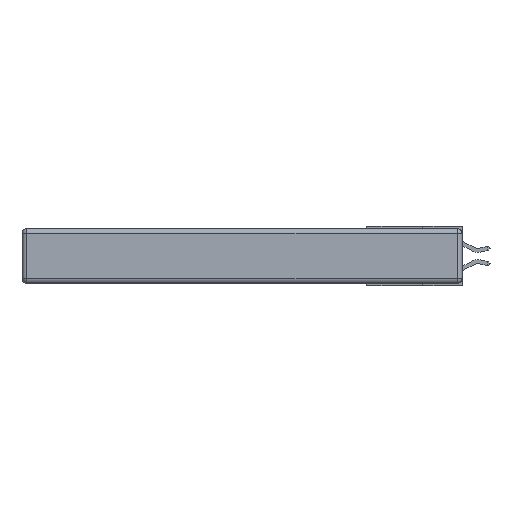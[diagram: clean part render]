
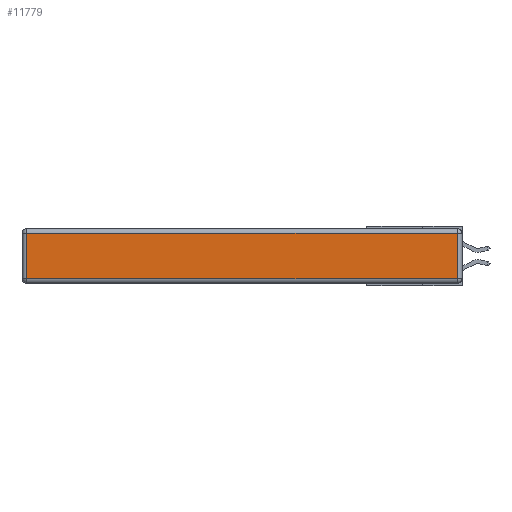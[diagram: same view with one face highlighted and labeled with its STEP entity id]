
A CAD part, left-side view. The second image highlights one B-rep face of the part: STEP entity #11779.
In plain terms, the highlighted planar face has unit normal (-1, 0, 0).
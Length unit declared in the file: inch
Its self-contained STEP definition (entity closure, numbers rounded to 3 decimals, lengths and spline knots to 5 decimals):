
#363 = CARTESIAN_POINT ( 'NONE',  ( 0., 2.72, -0.343 ) ) ;
#680 = ORIENTED_EDGE ( 'NONE', *, *, #1402, .T. ) ;
#689 = PLANE ( 'NONE',  #1484 ) ;
#889 = ORIENTED_EDGE ( 'NONE', *, *, #3025, .T. ) ;
#1402 = EDGE_CURVE ( 'NONE', #5856, #6088, #8198, .T. ) ;
#1484 = AXIS2_PLACEMENT_3D ( 'NONE', #8946, #13952, #6666 ) ;
#1620 = DIRECTION ( 'NONE',  ( 0., 0., -1. ) ) ;
#2012 = ORIENTED_EDGE ( 'NONE', *, *, #2764, .T. ) ;
#2402 = LINE ( 'NONE', #3396, #6455 ) ;
#2764 = EDGE_CURVE ( 'NONE', #6088, #13949, #13641, .T. ) ;
#3025 = EDGE_CURVE ( 'NONE', #13949, #10042, #5143, .T. ) ;
#3141 = VECTOR ( 'NONE', #4670, 39.37008 ) ;
#3396 = CARTESIAN_POINT ( 'NONE',  ( 0., 2.75, -0.03 ) ) ;
#3878 = CARTESIAN_POINT ( 'NONE',  ( 0., 0.03, -0.343 ) ) ;
#4144 = EDGE_LOOP ( 'NONE', ( #2012, #889, #14022, #680 ) ) ;
#4670 = DIRECTION ( 'NONE',  ( 0., -1., 0. ) ) ;
#5143 = LINE ( 'NONE', #3878, #15537 ) ;
#5577 = VECTOR ( 'NONE', #1620, 39.37008 ) ;
#5856 = VERTEX_POINT ( 'NONE', #15125 ) ;
#6088 = VERTEX_POINT ( 'NONE', #9663 ) ;
#6455 = VECTOR ( 'NONE', #14264, 39.37008 ) ;
#6666 = DIRECTION ( 'NONE',  ( 0., 0., 1. ) ) ;
#6733 = CARTESIAN_POINT ( 'NONE',  ( 0., 0.03, -0.03 ) ) ;
#8198 = LINE ( 'NONE', #363, #5577 ) ;
#8717 = FACE_OUTER_BOUND ( 'NONE', #4144, .T. ) ;
#8946 = CARTESIAN_POINT ( 'NONE',  ( 0., 0., -0.343 ) ) ;
#9548 = CARTESIAN_POINT ( 'NONE',  ( 0., 0., -0.313 ) ) ;
#9641 = CARTESIAN_POINT ( 'NONE',  ( 0., 0.03, -0.313 ) ) ;
#9663 = CARTESIAN_POINT ( 'NONE',  ( 0., 2.72, -0.313 ) ) ;
#9804 = DIRECTION ( 'NONE',  ( 0., 0., 1. ) ) ;
#10042 = VERTEX_POINT ( 'NONE', #6733 ) ;
#11779 = ADVANCED_FACE ( 'NONE', ( #8717 ), #689, .T. ) ;
#13641 = LINE ( 'NONE', #9548, #3141 ) ;
#13949 = VERTEX_POINT ( 'NONE', #9641 ) ;
#13952 = DIRECTION ( 'NONE',  ( -1., 0., 0. ) ) ;
#14022 = ORIENTED_EDGE ( 'NONE', *, *, #15086, .T. ) ;
#14264 = DIRECTION ( 'NONE',  ( 0., 1., 0. ) ) ;
#15086 = EDGE_CURVE ( 'NONE', #10042, #5856, #2402, .T. ) ;
#15125 = CARTESIAN_POINT ( 'NONE',  ( 0., 2.72, -0.03 ) ) ;
#15537 = VECTOR ( 'NONE', #9804, 39.37008 ) ;
